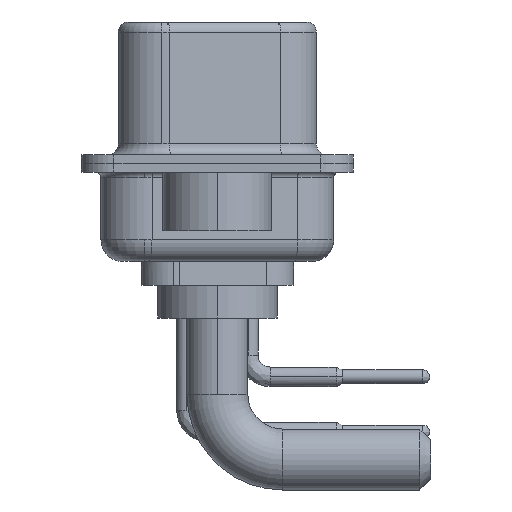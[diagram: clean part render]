
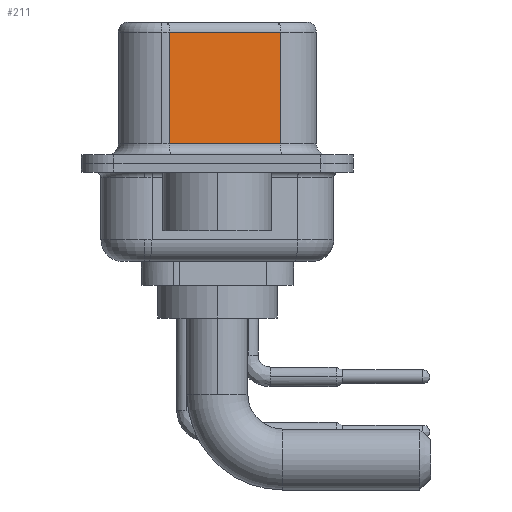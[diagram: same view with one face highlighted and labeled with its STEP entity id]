
A CAD part, left-side view. The second image highlights one B-rep face of the part: STEP entity #211.
In plain terms, the highlighted planar face has unit normal (-0.985, -0.174, 0).
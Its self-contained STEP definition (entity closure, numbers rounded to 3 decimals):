
#211 = ADVANCED_FACE ( 'NONE', ( #935 ), #11986, .F. ) ;
#807 = ORIENTED_EDGE ( 'NONE', *, *, #18562, .F. ) ;
#845 = LINE ( 'NONE', #20773, #16415 ) ;
#935 = FACE_OUTER_BOUND ( 'NONE', #17359, .T. ) ;
#1396 = DIRECTION ( 'NONE',  ( 0., 0., -1. ) ) ;
#3491 = ORIENTED_EDGE ( 'NONE', *, *, #24390, .T. ) ;
#4662 = LINE ( 'NONE', #21894, #8215 ) ;
#5528 = VECTOR ( 'NONE', #16671, 1000. ) ;
#5994 = VECTOR ( 'NONE', #24026, 1000. ) ;
#7025 = CARTESIAN_POINT ( 'NONE',  ( 4.58, -2.897, 0.9 ) ) ;
#7631 = CARTESIAN_POINT ( 'NONE',  ( 3.68, 2.203, 0.9 ) ) ;
#7883 = DIRECTION ( 'NONE',  ( -0.174, 0.985, 0. ) ) ;
#8215 = VECTOR ( 'NONE', #16614, 1000. ) ;
#10061 = LINE ( 'NONE', #14579, #5528 ) ;
#10216 = CARTESIAN_POINT ( 'NONE',  ( 4.58, -2.897, 6.02 ) ) ;
#10616 = VERTEX_POINT ( 'NONE', #10216 ) ;
#11597 = LINE ( 'NONE', #24303, #5994 ) ;
#11986 = PLANE ( 'NONE',  #19299 ) ;
#14579 = CARTESIAN_POINT ( 'NONE',  ( 3.68, 2.203, 6.52 ) ) ;
#16415 = VECTOR ( 'NONE', #1396, 1000. ) ;
#16614 = DIRECTION ( 'NONE',  ( 0.174, -0.985, 0. ) ) ;
#16671 = DIRECTION ( 'NONE',  ( 0., 0., -1. ) ) ;
#17359 = EDGE_LOOP ( 'NONE', ( #807, #3491, #24499, #22898 ) ) ;
#17818 = CARTESIAN_POINT ( 'NONE',  ( 3.68, 2.203, 6.02 ) ) ;
#18562 = EDGE_CURVE ( 'NONE', #10616, #24965, #845, .T. ) ;
#18647 = VERTEX_POINT ( 'NONE', #7631 ) ;
#19299 = AXIS2_PLACEMENT_3D ( 'NONE', #22563, #24975, #7883 ) ;
#20773 = CARTESIAN_POINT ( 'NONE',  ( 4.58, -2.897, 6.52 ) ) ;
#21894 = CARTESIAN_POINT ( 'NONE',  ( 4.58, -2.897, 0.9 ) ) ;
#22226 = EDGE_CURVE ( 'NONE', #18647, #24965, #4662, .T. ) ;
#22563 = CARTESIAN_POINT ( 'NONE',  ( 4.58, -2.897, 6.52 ) ) ;
#22898 = ORIENTED_EDGE ( 'NONE', *, *, #22226, .T. ) ;
#24026 = DIRECTION ( 'NONE',  ( -0.174, 0.985, 0. ) ) ;
#24056 = EDGE_CURVE ( 'NONE', #24263, #18647, #10061, .T. ) ;
#24263 = VERTEX_POINT ( 'NONE', #17818 ) ;
#24303 = CARTESIAN_POINT ( 'NONE',  ( 4.58, -2.897, 6.02 ) ) ;
#24390 = EDGE_CURVE ( 'NONE', #10616, #24263, #11597, .T. ) ;
#24499 = ORIENTED_EDGE ( 'NONE', *, *, #24056, .T. ) ;
#24965 = VERTEX_POINT ( 'NONE', #7025 ) ;
#24975 = DIRECTION ( 'NONE',  ( 0.985, 0.174, 0. ) ) ;
